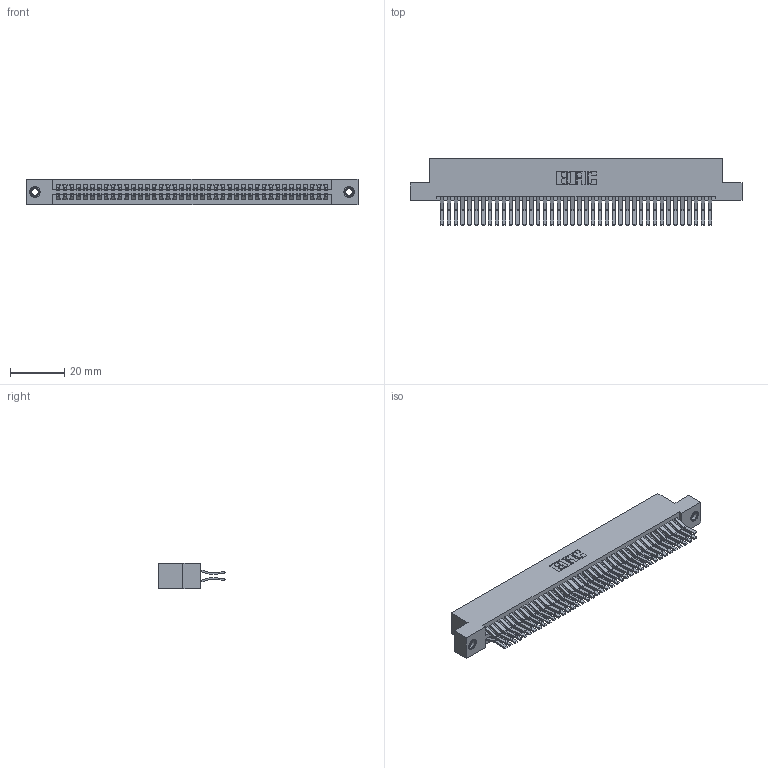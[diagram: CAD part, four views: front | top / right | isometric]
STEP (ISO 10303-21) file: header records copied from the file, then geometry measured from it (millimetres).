
FILE_DESCRIPTION (( 'STEP AP203' ), '1' );
FILE_NAME ('395-080-560-207.STEP', '2018-11-28T06:10:52', ( '' ), ( '' ), 'SwSTEP 2.0', 'SolidWorks 2016', '' );
FILE_SCHEMA (( 'CONFIG_CONTROL_DESIGN' ));
Length unit declared in the file: inch
Products named in the file (4): 345-250-001_345-250-005-103; 345-292-001_560 Tail; 345 Part_Flush Mounting Lugs - 0.156 Dia-TI; 395-080-560-207
Assembly tree (83 placements, depth 2):
  395-080-560-207
    345 Part_Flush Mounting Lugs - 0.156 Dia-TI
    345-292-001_560 Tail  x80
    345-250-001_345-250-005-103  x2
Bounding box: 122.81 x 24.45 x 9.4 mm (x, y, z)
Volume: 12422.1 mm3; surface area: 19699.7 mm2
Topology: 83 solids, 83 shells, 4346 faces, 12877 edges, 8470 vertices
Faces by surface type: plane 2752, cylinder 1578, cone 12, torus 4
Entity records: 32928 total; most frequent: CARTESIAN_POINT 5503, ORIENTED_EDGE 5430, DIRECTION 4885, EDGE_CURVE 2715, VECTOR 2399, LINE 2399, VERTEX_POINT 1804, AXIS2_PLACEMENT_3D 1243
